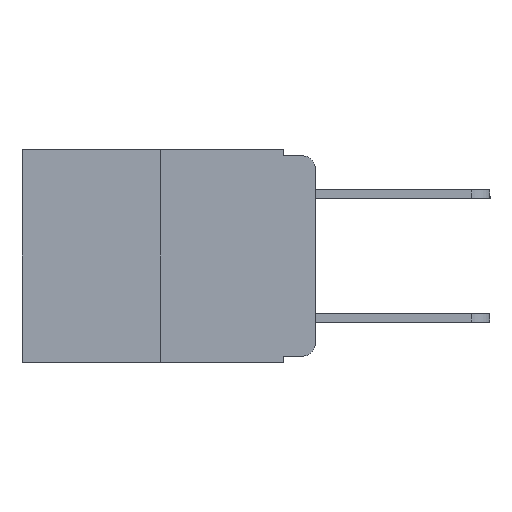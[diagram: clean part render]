
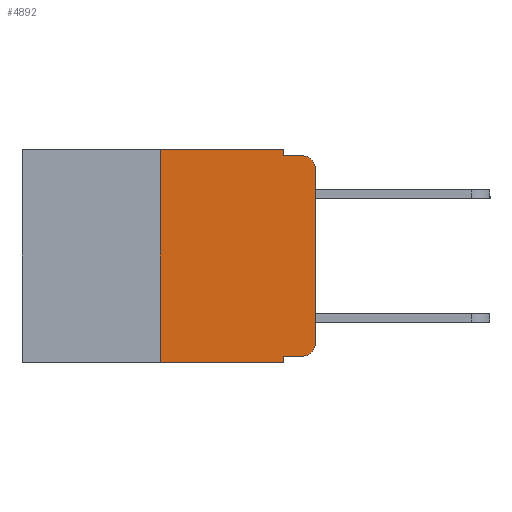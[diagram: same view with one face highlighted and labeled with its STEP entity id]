
A CAD part, left-side view. The second image highlights one B-rep face of the part: STEP entity #4892.
In plain terms, the highlighted planar face has unit normal (-1, 0, 0).
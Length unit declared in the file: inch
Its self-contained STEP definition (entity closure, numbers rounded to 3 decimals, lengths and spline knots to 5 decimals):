
#1192 = VECTOR ( 'NONE', #20820, 39.37008 ) ;
#1789 = DIRECTION ( 'NONE',  ( -1., 0., 0. ) ) ;
#1810 = CARTESIAN_POINT ( 'NONE',  ( 0., 0.051, -0.333 ) ) ;
#1982 = EDGE_CURVE ( 'NONE', #6687, #2490, #14251, .T. ) ;
#2429 = ORIENTED_EDGE ( 'NONE', *, *, #16049, .F. ) ;
#2490 = VERTEX_POINT ( 'NONE', #2764 ) ;
#2764 = CARTESIAN_POINT ( 'NONE',  ( 0., 0.02, -0.01 ) ) ;
#4012 = CARTESIAN_POINT ( 'NONE',  ( 0., 0.051, -0.01 ) ) ;
#4271 = AXIS2_PLACEMENT_3D ( 'NONE', #15312, #4698, #17057 ) ;
#4432 = EDGE_CURVE ( 'NONE', #13159, #20823, #14513, .T. ) ;
#4524 = FACE_OUTER_BOUND ( 'NONE', #17709, .T. ) ;
#4672 = VERTEX_POINT ( 'NONE', #13794 ) ;
#4680 = VERTEX_POINT ( 'NONE', #17914 ) ;
#4698 = DIRECTION ( 'NONE',  ( -1., 0., 0. ) ) ;
#4843 = LINE ( 'NONE', #1810, #19462 ) ;
#4892 = ADVANCED_FACE ( 'NONE', ( #4524 ), #12607, .F. ) ;
#5661 = CARTESIAN_POINT ( 'NONE',  ( 0., 0.051, -0.343 ) ) ;
#5745 = ORIENTED_EDGE ( 'NONE', *, *, #1982, .F. ) ;
#5764 = ORIENTED_EDGE ( 'NONE', *, *, #13195, .F. ) ;
#6543 = EDGE_CURVE ( 'NONE', #15854, #15860, #17680, .T. ) ;
#6629 = VERTEX_POINT ( 'NONE', #12439 ) ;
#6657 = CARTESIAN_POINT ( 'NONE',  ( 0., 0.051, 0. ) ) ;
#6687 = VERTEX_POINT ( 'NONE', #4012 ) ;
#7119 = DIRECTION ( 'NONE',  ( 0., -1., 0. ) ) ;
#8374 = AXIS2_PLACEMENT_3D ( 'NONE', #12371, #1789, #14129 ) ;
#8525 = ORIENTED_EDGE ( 'NONE', *, *, #22460, .F. ) ;
#9216 = DIRECTION ( 'NONE',  ( 0., -1., 0. ) ) ;
#9931 = ORIENTED_EDGE ( 'NONE', *, *, #6543, .T. ) ;
#10224 = VECTOR ( 'NONE', #21354, 39.37008 ) ;
#10363 = VECTOR ( 'NONE', #7119, 39.37008 ) ;
#10655 = CARTESIAN_POINT ( 'NONE',  ( 0., 0.25, 0. ) ) ;
#10749 = ORIENTED_EDGE ( 'NONE', *, *, #12027, .F. ) ;
#10775 = LINE ( 'NONE', #14421, #10224 ) ;
#11441 = EDGE_CURVE ( 'NONE', #6629, #2490, #17681, .T. ) ;
#11548 = CARTESIAN_POINT ( 'NONE',  ( 0., 0.02, -0.333 ) ) ;
#12027 = EDGE_CURVE ( 'NONE', #18065, #20823, #10775, .T. ) ;
#12083 = CARTESIAN_POINT ( 'NONE',  ( 0., 0.051, -0.333 ) ) ;
#12135 = CARTESIAN_POINT ( 'NONE',  ( 0., 0.051, -0.01 ) ) ;
#12371 = CARTESIAN_POINT ( 'NONE',  ( 0., 0.02, -0.313 ) ) ;
#12439 = CARTESIAN_POINT ( 'NONE',  ( 0., 0., -0.03 ) ) ;
#12607 = PLANE ( 'NONE',  #16895 ) ;
#13159 = VERTEX_POINT ( 'NONE', #17575 ) ;
#13188 = ORIENTED_EDGE ( 'NONE', *, *, #15020, .T. ) ;
#13195 = EDGE_CURVE ( 'NONE', #13159, #4672, #19553, .T. ) ;
#13515 = ORIENTED_EDGE ( 'NONE', *, *, #20664, .T. ) ;
#13794 = CARTESIAN_POINT ( 'NONE',  ( 0., 0.25, 0. ) ) ;
#13941 = CARTESIAN_POINT ( 'NONE',  ( 0., 0.473, 0. ) ) ;
#14070 = DIRECTION ( 'NONE',  ( 0., -1., 0. ) ) ;
#14087 = LINE ( 'NONE', #6657, #18198 ) ;
#14129 = DIRECTION ( 'NONE',  ( 0., 0., -1. ) ) ;
#14251 = LINE ( 'NONE', #12135, #22444 ) ;
#14347 = ORIENTED_EDGE ( 'NONE', *, *, #4432, .T. ) ;
#14356 = VECTOR ( 'NONE', #19417, 39.37008 ) ;
#14421 = CARTESIAN_POINT ( 'NONE',  ( 0., 0.051, 0. ) ) ;
#14461 = CARTESIAN_POINT ( 'NONE',  ( 0., 0., 0. ) ) ;
#14513 = LINE ( 'NONE', #18973, #10363 ) ;
#14742 = LINE ( 'NONE', #13941, #1192 ) ;
#15020 = EDGE_CURVE ( 'NONE', #15860, #6629, #18366, .T. ) ;
#15127 = CARTESIAN_POINT ( 'NONE',  ( 0., 0., -0.313 ) ) ;
#15170 = DIRECTION ( 'NONE',  ( 0., 0., -1. ) ) ;
#15312 = CARTESIAN_POINT ( 'NONE',  ( 0., 0.02, -0.03 ) ) ;
#15854 = VERTEX_POINT ( 'NONE', #11548 ) ;
#15860 = VERTEX_POINT ( 'NONE', #15127 ) ;
#16049 = EDGE_CURVE ( 'NONE', #4672, #4680, #14742, .T. ) ;
#16228 = DIRECTION ( 'NONE',  ( 0., 0., 1. ) ) ;
#16895 = AXIS2_PLACEMENT_3D ( 'NONE', #19154, #17439, #15170 ) ;
#17057 = DIRECTION ( 'NONE',  ( 0., 0., -1. ) ) ;
#17294 = DIRECTION ( 'NONE',  ( 0., 0., -1. ) ) ;
#17439 = DIRECTION ( 'NONE',  ( 1., 0., 0. ) ) ;
#17575 = CARTESIAN_POINT ( 'NONE',  ( 0., 0.25, -0.343 ) ) ;
#17680 = CIRCLE ( 'NONE', #8374, 0.02 ) ;
#17681 = CIRCLE ( 'NONE', #4271, 0.02 ) ;
#17709 = EDGE_LOOP ( 'NONE', ( #13188, #20587, #5745, #8525, #2429, #5764, #14347, #10749, #13515, #9931 ) ) ;
#17832 = VECTOR ( 'NONE', #16228, 39.37008 ) ;
#17914 = CARTESIAN_POINT ( 'NONE',  ( 0., 0.051, 0. ) ) ;
#18065 = VERTEX_POINT ( 'NONE', #12083 ) ;
#18198 = VECTOR ( 'NONE', #17294, 39.37008 ) ;
#18366 = LINE ( 'NONE', #14461, #17832 ) ;
#18973 = CARTESIAN_POINT ( 'NONE',  ( 0., 0.473, -0.343 ) ) ;
#19154 = CARTESIAN_POINT ( 'NONE',  ( 0., 0.473, 0. ) ) ;
#19417 = DIRECTION ( 'NONE',  ( 0., 0., 1. ) ) ;
#19462 = VECTOR ( 'NONE', #14070, 39.37008 ) ;
#19553 = LINE ( 'NONE', #10655, #14356 ) ;
#20587 = ORIENTED_EDGE ( 'NONE', *, *, #11441, .T. ) ;
#20664 = EDGE_CURVE ( 'NONE', #18065, #15854, #4843, .T. ) ;
#20820 = DIRECTION ( 'NONE',  ( 0., -1., 0. ) ) ;
#20823 = VERTEX_POINT ( 'NONE', #5661 ) ;
#21354 = DIRECTION ( 'NONE',  ( 0., 0., -1. ) ) ;
#22444 = VECTOR ( 'NONE', #9216, 39.37008 ) ;
#22460 = EDGE_CURVE ( 'NONE', #4680, #6687, #14087, .T. ) ;
